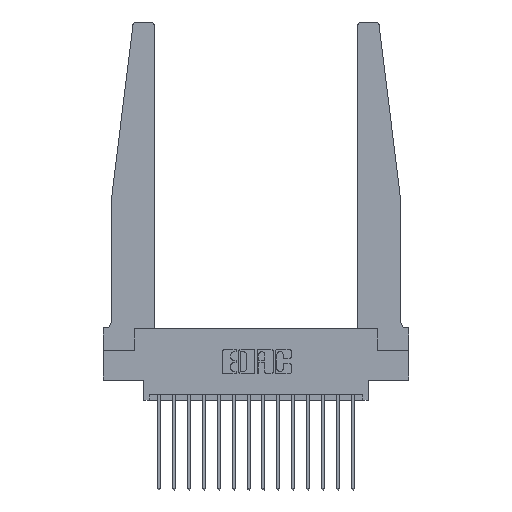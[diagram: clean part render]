
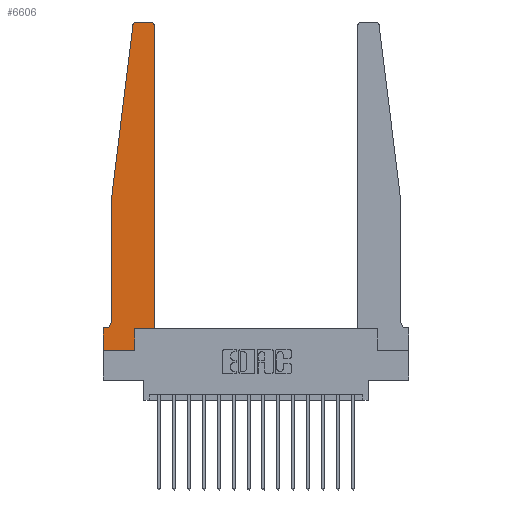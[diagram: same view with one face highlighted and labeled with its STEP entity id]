
A CAD part, top view. The second image highlights one B-rep face of the part: STEP entity #6606.
In plain terms, the highlighted planar face has unit normal (0, 0, 1).
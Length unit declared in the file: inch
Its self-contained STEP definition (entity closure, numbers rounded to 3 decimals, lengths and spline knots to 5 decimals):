
#91 = VERTEX_POINT ( 'NONE', #6720 ) ;
#166 = EDGE_CURVE ( 'NONE', #91, #17665, #2910, .T. ) ;
#366 = VECTOR ( 'NONE', #14346, 39.37008 ) ;
#636 = EDGE_CURVE ( 'NONE', #15205, #18128, #14717, .T. ) ;
#642 = EDGE_CURVE ( 'NONE', #18128, #11788, #675, .T. ) ;
#644 = AXIS2_PLACEMENT_3D ( 'NONE', #10464, #3464, #3097 ) ;
#665 = DIRECTION ( 'NONE',  ( 0., 1., 0. ) ) ;
#675 = CIRCLE ( 'NONE', #1858, 0.03 ) ;
#717 = CARTESIAN_POINT ( 'NONE',  ( 0., 0., 0.37 ) ) ;
#834 = ORIENTED_EDGE ( 'NONE', *, *, #166, .T. ) ;
#946 = VERTEX_POINT ( 'NONE', #2582 ) ;
#1054 = VERTEX_POINT ( 'NONE', #9243 ) ;
#1261 = CIRCLE ( 'NONE', #11558, 0.03 ) ;
#1364 = VERTEX_POINT ( 'NONE', #717 ) ;
#1690 = EDGE_CURVE ( 'NONE', #1364, #11324, #2052, .T. ) ;
#1726 = ORIENTED_EDGE ( 'NONE', *, *, #642, .T. ) ;
#1775 = DIRECTION ( 'NONE',  ( 0., 0., 1. ) ) ;
#1858 = AXIS2_PLACEMENT_3D ( 'NONE', #3167, #1775, #13062 ) ;
#2006 = CARTESIAN_POINT ( 'NONE',  ( 0.27653, 2.75, 0.37 ) ) ;
#2052 = LINE ( 'NONE', #6332, #4061 ) ;
#2144 = DIRECTION ( 'NONE',  ( 0., 1., 0. ) ) ;
#2582 = CARTESIAN_POINT ( 'NONE',  ( 0.425, 2.72, 0.37 ) ) ;
#2910 = LINE ( 'NONE', #12600, #3367 ) ;
#2978 = LINE ( 'NONE', #3163, #7957 ) ;
#3097 = DIRECTION ( 'NONE',  ( 1., 0., 0. ) ) ;
#3110 = CARTESIAN_POINT ( 'NONE',  ( 0., 0.1875, 0.37 ) ) ;
#3163 = CARTESIAN_POINT ( 'NONE',  ( 0.065, 1.25, 0.37 ) ) ;
#3167 = CARTESIAN_POINT ( 'NONE',  ( 0.27653, 2.72, 0.37 ) ) ;
#3217 = ORIENTED_EDGE ( 'NONE', *, *, #15638, .T. ) ;
#3260 = CARTESIAN_POINT ( 'NONE',  ( 0.065, 1.25, 0.37 ) ) ;
#3367 = VECTOR ( 'NONE', #14187, 39.37008 ) ;
#3443 = CARTESIAN_POINT ( 'NONE',  ( 0.065, 0.2375, 0.37 ) ) ;
#3464 = DIRECTION ( 'NONE',  ( 0., 0., 1. ) ) ;
#3466 = DIRECTION ( 'NONE',  ( 1., 0., 0. ) ) ;
#3556 = LINE ( 'NONE', #7891, #13518 ) ;
#3608 = EDGE_CURVE ( 'NONE', #11788, #1054, #17401, .T. ) ;
#3763 = FACE_OUTER_BOUND ( 'NONE', #6061, .T. ) ;
#4061 = VECTOR ( 'NONE', #3466, 39.37008 ) ;
#4065 = VERTEX_POINT ( 'NONE', #3110 ) ;
#4331 = DIRECTION ( 'NONE',  ( 0., -1., 0. ) ) ;
#4380 = ORIENTED_EDGE ( 'NONE', *, *, #16976, .T. ) ;
#4548 = VECTOR ( 'NONE', #8677, 39.37008 ) ;
#4563 = EDGE_CURVE ( 'NONE', #946, #15205, #1261, .T. ) ;
#4625 = EDGE_CURVE ( 'NONE', #4811, #4065, #13847, .T. ) ;
#4811 = VERTEX_POINT ( 'NONE', #15379 ) ;
#4878 = CARTESIAN_POINT ( 'NONE',  ( 0.24675, 2.72367, 0.37 ) ) ;
#5140 = ORIENTED_EDGE ( 'NONE', *, *, #636, .T. ) ;
#5242 = PLANE ( 'NONE',  #644 ) ;
#5351 = LINE ( 'NONE', #16866, #10185 ) ;
#5544 = ORIENTED_EDGE ( 'NONE', *, *, #10954, .T. ) ;
#5680 = DIRECTION ( 'NONE',  ( 0., -1., 0. ) ) ;
#5871 = CARTESIAN_POINT ( 'NONE',  ( 0.25, 2.75, 0.37 ) ) ;
#6061 = EDGE_LOOP ( 'NONE', ( #5140, #1726, #11956, #4380, #3217, #13078, #5544, #7114, #11584, #834, #16181, #10373 ) ) ;
#6282 = CARTESIAN_POINT ( 'NONE',  ( 0.395, 2.75, 0.37 ) ) ;
#6332 = CARTESIAN_POINT ( 'NONE',  ( 0., 0., 0.37 ) ) ;
#6606 = ADVANCED_FACE ( 'NONE', ( #3763 ), #5242, .T. ) ;
#6720 = CARTESIAN_POINT ( 'NONE',  ( 0.2605, 0.18, 0.37 ) ) ;
#7114 = ORIENTED_EDGE ( 'NONE', *, *, #1690, .T. ) ;
#7891 = CARTESIAN_POINT ( 'NONE',  ( 0.2605, 0.18, 0.37 ) ) ;
#7957 = VECTOR ( 'NONE', #5680, 39.37008 ) ;
#8512 = AXIS2_PLACEMENT_3D ( 'NONE', #15274, #11014, #18244 ) ;
#8677 = DIRECTION ( 'NONE',  ( -1., 0., 0. ) ) ;
#8904 = DIRECTION ( 'NONE',  ( -0.122, -0.992, 0. ) ) ;
#9243 = CARTESIAN_POINT ( 'NONE',  ( 0.065, 1.25, 0.37 ) ) ;
#9389 = CARTESIAN_POINT ( 'NONE',  ( 0.425, 0.18, 0.37 ) ) ;
#9786 = EDGE_CURVE ( 'NONE', #17665, #946, #14707, .T. ) ;
#9981 = DIRECTION ( 'NONE',  ( 0., 0., 1. ) ) ;
#10185 = VECTOR ( 'NONE', #4331, 39.37008 ) ;
#10373 = ORIENTED_EDGE ( 'NONE', *, *, #4563, .T. ) ;
#10464 = CARTESIAN_POINT ( 'NONE',  ( 0., 0.1875, 0.37 ) ) ;
#10776 = CARTESIAN_POINT ( 'NONE',  ( 0.2605, 0., 0.37 ) ) ;
#10954 = EDGE_CURVE ( 'NONE', #4065, #1364, #5351, .T. ) ;
#11014 = DIRECTION ( 'NONE',  ( 0., 0., -1. ) ) ;
#11034 = VECTOR ( 'NONE', #2144, 39.37008 ) ;
#11324 = VERTEX_POINT ( 'NONE', #10776 ) ;
#11517 = VERTEX_POINT ( 'NONE', #3443 ) ;
#11558 = AXIS2_PLACEMENT_3D ( 'NONE', #14149, #9981, #12753 ) ;
#11584 = ORIENTED_EDGE ( 'NONE', *, *, #15869, .T. ) ;
#11788 = VERTEX_POINT ( 'NONE', #4878 ) ;
#11956 = ORIENTED_EDGE ( 'NONE', *, *, #3608, .T. ) ;
#12600 = CARTESIAN_POINT ( 'NONE',  ( 0.425, 0.18, 0.37 ) ) ;
#12753 = DIRECTION ( 'NONE',  ( 1., 0., 0. ) ) ;
#12924 = CARTESIAN_POINT ( 'NONE',  ( 0.065, 0.1875, 0.37 ) ) ;
#13062 = DIRECTION ( 'NONE',  ( 1., 0., 0. ) ) ;
#13078 = ORIENTED_EDGE ( 'NONE', *, *, #4625, .T. ) ;
#13518 = VECTOR ( 'NONE', #665, 39.37008 ) ;
#13847 = LINE ( 'NONE', #12924, #4548 ) ;
#14149 = CARTESIAN_POINT ( 'NONE',  ( 0.395, 2.72, 0.37 ) ) ;
#14187 = DIRECTION ( 'NONE',  ( 1., 0., 0. ) ) ;
#14346 = DIRECTION ( 'NONE',  ( -1., 0., 0. ) ) ;
#14707 = LINE ( 'NONE', #17595, #11034 ) ;
#14717 = LINE ( 'NONE', #5871, #366 ) ;
#15205 = VERTEX_POINT ( 'NONE', #6282 ) ;
#15274 = CARTESIAN_POINT ( 'NONE',  ( 0.015, 0.2375, 0.37 ) ) ;
#15379 = CARTESIAN_POINT ( 'NONE',  ( 0.015, 0.1875, 0.37 ) ) ;
#15633 = VECTOR ( 'NONE', #8904, 39.37008 ) ;
#15638 = EDGE_CURVE ( 'NONE', #11517, #4811, #15857, .T. ) ;
#15857 = CIRCLE ( 'NONE', #8512, 0.05 ) ;
#15869 = EDGE_CURVE ( 'NONE', #11324, #91, #3556, .T. ) ;
#16181 = ORIENTED_EDGE ( 'NONE', *, *, #9786, .T. ) ;
#16866 = CARTESIAN_POINT ( 'NONE',  ( 0., 0., 0.37 ) ) ;
#16976 = EDGE_CURVE ( 'NONE', #1054, #11517, #2978, .T. ) ;
#17401 = LINE ( 'NONE', #3260, #15633 ) ;
#17595 = CARTESIAN_POINT ( 'NONE',  ( 0.425, 0.18, 0.37 ) ) ;
#17665 = VERTEX_POINT ( 'NONE', #9389 ) ;
#18128 = VERTEX_POINT ( 'NONE', #2006 ) ;
#18244 = DIRECTION ( 'NONE',  ( -1., 0., 0. ) ) ;
